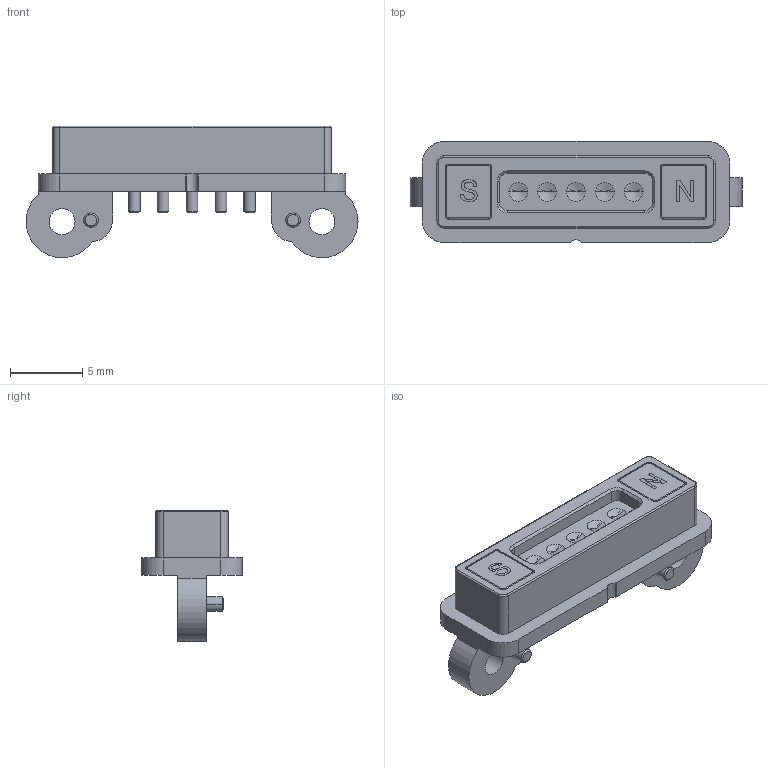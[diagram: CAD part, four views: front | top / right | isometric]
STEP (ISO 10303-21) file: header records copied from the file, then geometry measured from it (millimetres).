
FILE_DESCRIPTION (( 'STEP AP203' ), '1' );
FILE_NAME ('686-J0521250124.STEP', '2023-02-03T17:05:38', ( 'Magnum' ), ( '' ), 'SwSTEP 2.0', 'SolidWorks 2020', '' );
FILE_SCHEMA (( 'CONFIG_CONTROL_DESIGN' ));
Length unit declared in the file: millimetre
Products named in the file (1): 686-J0521250124
Bounding box: 23 x 7 x 9.1 mm (x, y, z)
Volume: 515.7 mm3; surface area: 809.3 mm2
Topology: 1 solids, 3 shells, 228 faces, 561 edges, 348 vertices
Faces by surface type: plane 83, cylinder 74, cone 37, bspline 26, torus 8
Entity records: 7697 total; most frequent: CARTESIAN_POINT 2270, DIRECTION 1122, ORIENTED_EDGE 1102, EDGE_CURVE 551, AXIS2_PLACEMENT_3D 408, VERTEX_POINT 348, VECTOR 306, LINE 306
